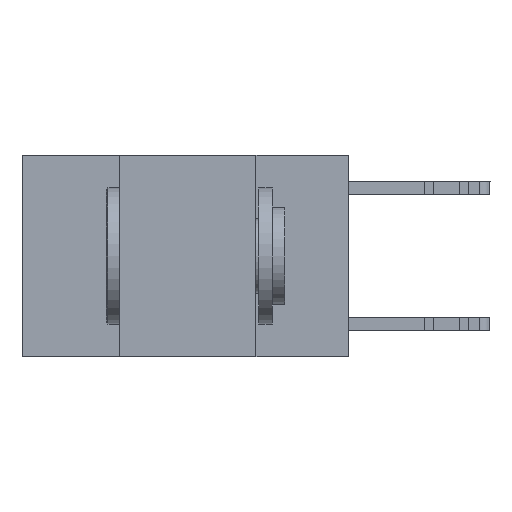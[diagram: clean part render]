
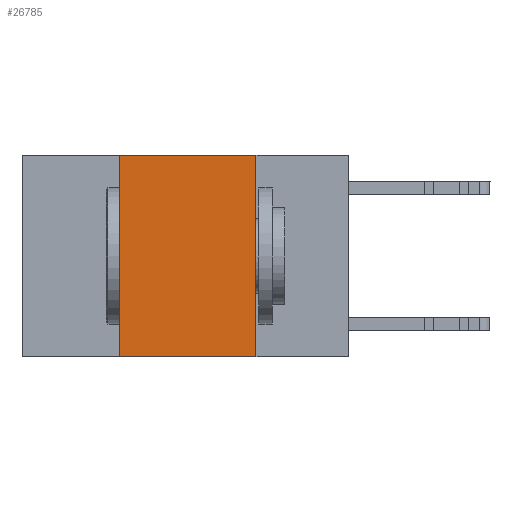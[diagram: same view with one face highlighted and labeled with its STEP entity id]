
A CAD part, left-side view. The second image highlights one B-rep face of the part: STEP entity #26785.
In plain terms, the highlighted planar face has unit normal (-1, 0, 0).
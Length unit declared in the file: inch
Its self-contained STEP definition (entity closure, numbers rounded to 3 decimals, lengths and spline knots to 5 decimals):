
#728 = EDGE_CURVE ( 'NONE', #10220, #14238, #12546, .T. ) ;
#791 = ORIENTED_EDGE ( 'NONE', *, *, #11072, .F. ) ;
#1265 = FACE_OUTER_BOUND ( 'NONE', #18892, .T. ) ;
#2948 = ORIENTED_EDGE ( 'NONE', *, *, #8660, .T. ) ;
#4117 = DIRECTION ( 'NONE',  ( 1., 0., 0. ) ) ;
#5138 = DIRECTION ( 'NONE',  ( 0., 0., 1. ) ) ;
#5228 = VECTOR ( 'NONE', #17682, 39.37008 ) ;
#5372 = CARTESIAN_POINT ( 'NONE',  ( 0., 0.6, 0. ) ) ;
#6238 = CARTESIAN_POINT ( 'NONE',  ( 0., 0.6, -0.37 ) ) ;
#7284 = LINE ( 'NONE', #5372, #10358 ) ;
#7445 = EDGE_CURVE ( 'NONE', #16471, #10220, #7284, .T. ) ;
#8660 = EDGE_CURVE ( 'NONE', #28466, #14238, #16374, .T. ) ;
#10220 = VERTEX_POINT ( 'NONE', #25966 ) ;
#10358 = VECTOR ( 'NONE', #17271, 39.37008 ) ;
#10966 = VECTOR ( 'NONE', #5138, 39.37008 ) ;
#11072 = EDGE_CURVE ( 'NONE', #28466, #16471, #22457, .T. ) ;
#11200 = DIRECTION ( 'NONE',  ( 0., 0., -1. ) ) ;
#11518 = CARTESIAN_POINT ( 'NONE',  ( 0., 0.6, 0. ) ) ;
#12546 = LINE ( 'NONE', #22321, #5228 ) ;
#14016 = AXIS2_PLACEMENT_3D ( 'NONE', #11518, #4117, #11200 ) ;
#14238 = VERTEX_POINT ( 'NONE', #23081 ) ;
#15870 = PLANE ( 'NONE',  #14016 ) ;
#16374 = LINE ( 'NONE', #6238, #25296 ) ;
#16471 = VERTEX_POINT ( 'NONE', #28030 ) ;
#17271 = DIRECTION ( 'NONE',  ( 0., -1., 0. ) ) ;
#17682 = DIRECTION ( 'NONE',  ( 0., 0., -1. ) ) ;
#18892 = EDGE_LOOP ( 'NONE', ( #25309, #23943, #791, #2948 ) ) ;
#22321 = CARTESIAN_POINT ( 'NONE',  ( 0., 0.17, 0. ) ) ;
#22457 = LINE ( 'NONE', #25196, #10966 ) ;
#23081 = CARTESIAN_POINT ( 'NONE',  ( 0., 0.17, -0.37 ) ) ;
#23943 = ORIENTED_EDGE ( 'NONE', *, *, #7445, .F. ) ;
#23969 = CARTESIAN_POINT ( 'NONE',  ( 0., 0.42, -0.37 ) ) ;
#25196 = CARTESIAN_POINT ( 'NONE',  ( 0., 0.42, 0. ) ) ;
#25296 = VECTOR ( 'NONE', #25842, 39.37008 ) ;
#25309 = ORIENTED_EDGE ( 'NONE', *, *, #728, .F. ) ;
#25842 = DIRECTION ( 'NONE',  ( 0., -1., 0. ) ) ;
#25966 = CARTESIAN_POINT ( 'NONE',  ( 0., 0.17, 0. ) ) ;
#26785 = ADVANCED_FACE ( 'NONE', ( #1265 ), #15870, .F. ) ;
#28030 = CARTESIAN_POINT ( 'NONE',  ( 0., 0.42, 0. ) ) ;
#28466 = VERTEX_POINT ( 'NONE', #23969 ) ;
